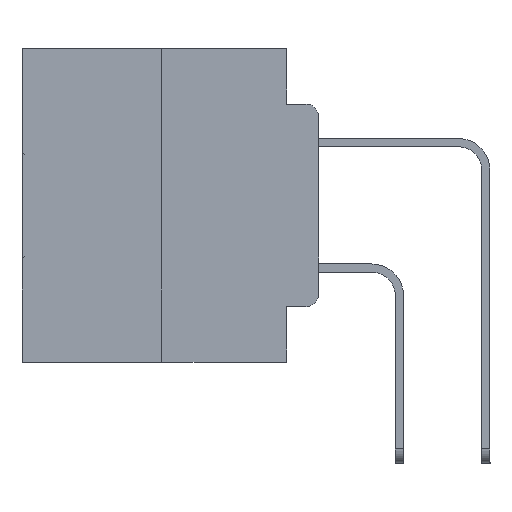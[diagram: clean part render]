
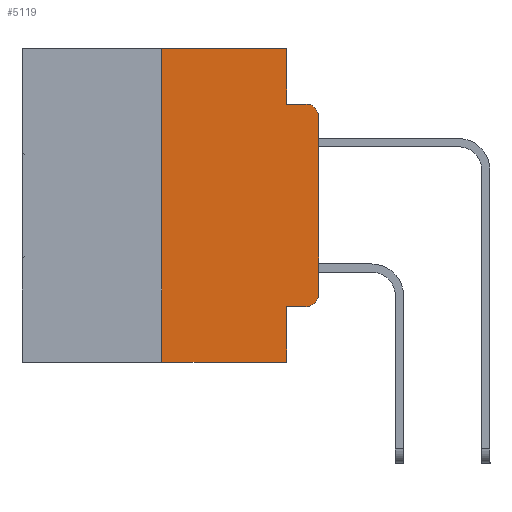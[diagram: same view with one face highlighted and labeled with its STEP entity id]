
A CAD part, left-side view. The second image highlights one B-rep face of the part: STEP entity #5119.
In plain terms, the highlighted planar face has unit normal (-1, 0, 0).
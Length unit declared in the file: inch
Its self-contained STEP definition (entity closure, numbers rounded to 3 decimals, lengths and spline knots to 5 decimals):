
#895 = ORIENTED_EDGE ( 'NONE', *, *, #10326, .F. ) ;
#1094 = DIRECTION ( 'NONE',  ( 0., 0., -1. ) ) ;
#1648 = EDGE_CURVE ( 'NONE', #29251, #5375, #22960, .T. ) ;
#2569 = CARTESIAN_POINT ( 'NONE',  ( 0., 0., -0.3915 ) ) ;
#2633 = CARTESIAN_POINT ( 'NONE',  ( 0., 0.051, -0.4115 ) ) ;
#3667 = CARTESIAN_POINT ( 'NONE',  ( 0., 0.02, -0.1085 ) ) ;
#4456 = EDGE_CURVE ( 'NONE', #5238, #24334, #16866, .T. ) ;
#4659 = ORIENTED_EDGE ( 'NONE', *, *, #33046, .F. ) ;
#4789 = CARTESIAN_POINT ( 'NONE',  ( 0., 0., 0. ) ) ;
#4807 = DIRECTION ( 'NONE',  ( 0., -1., 0. ) ) ;
#5036 = DIRECTION ( 'NONE',  ( 0., 0., -1. ) ) ;
#5119 = ADVANCED_FACE ( 'NONE', ( #9686 ), #27807, .F. ) ;
#5238 = VERTEX_POINT ( 'NONE', #2569 ) ;
#5257 = ORIENTED_EDGE ( 'NONE', *, *, #22899, .T. ) ;
#5375 = VERTEX_POINT ( 'NONE', #31285 ) ;
#5489 = VERTEX_POINT ( 'NONE', #6206 ) ;
#5714 = ORIENTED_EDGE ( 'NONE', *, *, #23955, .T. ) ;
#6206 = CARTESIAN_POINT ( 'NONE',  ( 0., 0.02, -0.4115 ) ) ;
#6276 = DIRECTION ( 'NONE',  ( 0., 0., -1. ) ) ;
#6563 = DIRECTION ( 'NONE',  ( 0., -1., 0. ) ) ;
#7185 = VECTOR ( 'NONE', #5036, 39.37008 ) ;
#7881 = CARTESIAN_POINT ( 'NONE',  ( 0., 0.051, -0.0885 ) ) ;
#7900 = VERTEX_POINT ( 'NONE', #2633 ) ;
#7956 = EDGE_CURVE ( 'NONE', #15055, #10858, #14650, .T. ) ;
#9686 = FACE_OUTER_BOUND ( 'NONE', #29586, .T. ) ;
#10242 = VECTOR ( 'NONE', #1094, 39.37008 ) ;
#10247 = LINE ( 'NONE', #20142, #31302 ) ;
#10326 = EDGE_CURVE ( 'NONE', #29251, #15055, #13359, .T. ) ;
#10800 = CARTESIAN_POINT ( 'NONE',  ( 0., 0.051, 0. ) ) ;
#10838 = CARTESIAN_POINT ( 'NONE',  ( 0., 0.473, -0.5 ) ) ;
#10858 = VERTEX_POINT ( 'NONE', #10800 ) ;
#11750 = VECTOR ( 'NONE', #22708, 39.37008 ) ;
#12068 = EDGE_CURVE ( 'NONE', #10858, #16652, #14009, .T. ) ;
#12737 = CARTESIAN_POINT ( 'NONE',  ( 0., 0.051, 0. ) ) ;
#13068 = VECTOR ( 'NONE', #28399, 39.37008 ) ;
#13359 = LINE ( 'NONE', #28612, #32798 ) ;
#14009 = LINE ( 'NONE', #12737, #7185 ) ;
#14650 = LINE ( 'NONE', #25821, #13068 ) ;
#15055 = VERTEX_POINT ( 'NONE', #23192 ) ;
#15077 = DIRECTION ( 'NONE',  ( 1., 0., 0. ) ) ;
#15089 = CARTESIAN_POINT ( 'NONE',  ( 0., 0.02, -0.3915 ) ) ;
#16158 = VECTOR ( 'NONE', #20559, 39.37008 ) ;
#16652 = VERTEX_POINT ( 'NONE', #7881 ) ;
#16844 = CARTESIAN_POINT ( 'NONE',  ( 0., 0.051, -0.4115 ) ) ;
#16866 = LINE ( 'NONE', #4789, #11750 ) ;
#17047 = ORIENTED_EDGE ( 'NONE', *, *, #1648, .T. ) ;
#17348 = ORIENTED_EDGE ( 'NONE', *, *, #12068, .F. ) ;
#17641 = DIRECTION ( 'NONE',  ( 0., 0., -1. ) ) ;
#18969 = CARTESIAN_POINT ( 'NONE',  ( 0., 0.051, 0. ) ) ;
#20142 = CARTESIAN_POINT ( 'NONE',  ( 0., 0.051, -0.0885 ) ) ;
#20215 = AXIS2_PLACEMENT_3D ( 'NONE', #30326, #15077, #32832 ) ;
#20559 = DIRECTION ( 'NONE',  ( 0., -1., 0. ) ) ;
#21040 = DIRECTION ( 'NONE',  ( 0., 0., 1. ) ) ;
#21164 = CARTESIAN_POINT ( 'NONE',  ( 0., 0., -0.1085 ) ) ;
#21618 = DIRECTION ( 'NONE',  ( -1., 0., 0. ) ) ;
#22269 = EDGE_CURVE ( 'NONE', #16652, #29496, #10247, .T. ) ;
#22708 = DIRECTION ( 'NONE',  ( 0., 0., 1. ) ) ;
#22899 = EDGE_CURVE ( 'NONE', #5489, #5238, #27234, .T. ) ;
#22960 = LINE ( 'NONE', #10838, #16158 ) ;
#23192 = CARTESIAN_POINT ( 'NONE',  ( 0., 0.25, 0. ) ) ;
#23757 = LINE ( 'NONE', #18969, #10242 ) ;
#23831 = CARTESIAN_POINT ( 'NONE',  ( 0., 0.25, -0.5 ) ) ;
#23955 = EDGE_CURVE ( 'NONE', #24334, #29496, #29935, .T. ) ;
#24334 = VERTEX_POINT ( 'NONE', #21164 ) ;
#24711 = ORIENTED_EDGE ( 'NONE', *, *, #7956, .F. ) ;
#25821 = CARTESIAN_POINT ( 'NONE',  ( 0., 0.473, 0. ) ) ;
#26211 = VECTOR ( 'NONE', #6563, 39.37008 ) ;
#26355 = ORIENTED_EDGE ( 'NONE', *, *, #4456, .T. ) ;
#27234 = CIRCLE ( 'NONE', #31631, 0.02 ) ;
#27807 = PLANE ( 'NONE',  #20215 ) ;
#28399 = DIRECTION ( 'NONE',  ( 0., -1., 0. ) ) ;
#28612 = CARTESIAN_POINT ( 'NONE',  ( 0., 0.25, 0. ) ) ;
#29251 = VERTEX_POINT ( 'NONE', #23831 ) ;
#29496 = VERTEX_POINT ( 'NONE', #30482 ) ;
#29586 = EDGE_LOOP ( 'NONE', ( #26355, #5714, #29973, #17348, #24711, #895, #17047, #4659, #32875, #5257 ) ) ;
#29935 = CIRCLE ( 'NONE', #31433, 0.02 ) ;
#29973 = ORIENTED_EDGE ( 'NONE', *, *, #22269, .F. ) ;
#30326 = CARTESIAN_POINT ( 'NONE',  ( 0., 0.473, 0. ) ) ;
#30482 = CARTESIAN_POINT ( 'NONE',  ( 0., 0.02, -0.0885 ) ) ;
#31285 = CARTESIAN_POINT ( 'NONE',  ( 0., 0.051, -0.5 ) ) ;
#31302 = VECTOR ( 'NONE', #4807, 39.37008 ) ;
#31380 = EDGE_CURVE ( 'NONE', #7900, #5489, #32146, .T. ) ;
#31433 = AXIS2_PLACEMENT_3D ( 'NONE', #3667, #21618, #6276 ) ;
#31631 = AXIS2_PLACEMENT_3D ( 'NONE', #15089, #32843, #17641 ) ;
#32146 = LINE ( 'NONE', #16844, #26211 ) ;
#32798 = VECTOR ( 'NONE', #21040, 39.37008 ) ;
#32832 = DIRECTION ( 'NONE',  ( 0., 0., -1. ) ) ;
#32843 = DIRECTION ( 'NONE',  ( -1., 0., 0. ) ) ;
#32875 = ORIENTED_EDGE ( 'NONE', *, *, #31380, .T. ) ;
#33046 = EDGE_CURVE ( 'NONE', #7900, #5375, #23757, .T. ) ;
